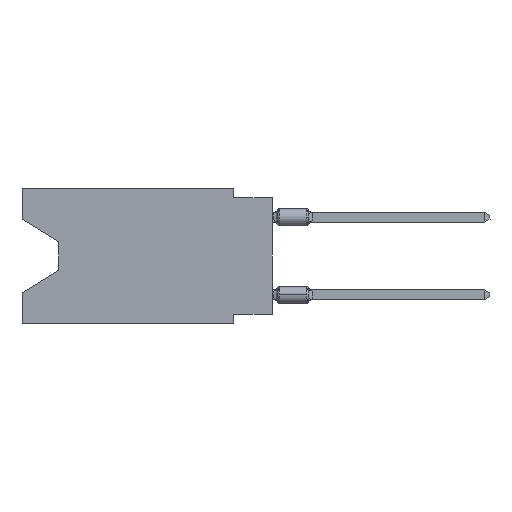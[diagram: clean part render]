
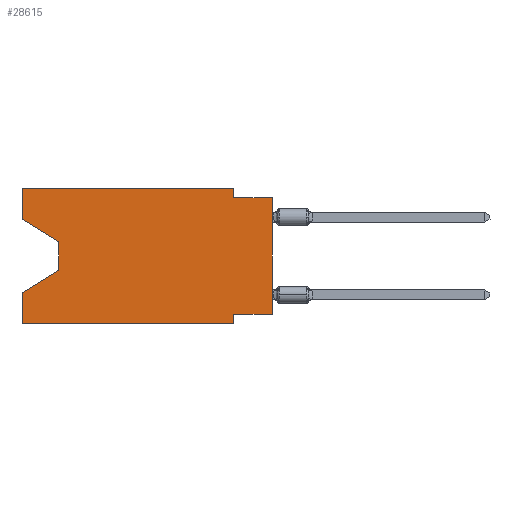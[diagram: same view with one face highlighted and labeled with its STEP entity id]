
A CAD part, left-side view. The second image highlights one B-rep face of the part: STEP entity #28615.
In plain terms, the highlighted planar face has unit normal (-1, 0, 0).
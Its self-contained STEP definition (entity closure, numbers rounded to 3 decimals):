
#139 = VERTEX_POINT ( 'NONE', #449 ) ;
#225 = DIRECTION ( 'NONE',  ( 0., 0.855, -0.519 ) ) ;
#449 = CARTESIAN_POINT ( 'NONE',  ( 0., 2.54, 0. ) ) ;
#458 = LINE ( 'NONE', #601, #13027 ) ;
#601 = CARTESIAN_POINT ( 'NONE',  ( 0., 2.54, -8.89 ) ) ;
#756 = VERTEX_POINT ( 'NONE', #26318 ) ;
#766 = DIRECTION ( 'NONE',  ( 0., -1., 0. ) ) ;
#1188 = CARTESIAN_POINT ( 'NONE',  ( 0., 16.383, -8.89 ) ) ;
#1565 = EDGE_CURVE ( 'NONE', #23276, #14872, #20340, .T. ) ;
#2100 = DIRECTION ( 'NONE',  ( 0., -1., 0. ) ) ;
#2121 = ORIENTED_EDGE ( 'NONE', *, *, #10918, .T. ) ;
#2343 = EDGE_LOOP ( 'NONE', ( #24505, #21543, #2121, #18915, #24399, #26511, #4750, #2411, #23506, #7458, #22411, #13040 ) ) ;
#2411 = ORIENTED_EDGE ( 'NONE', *, *, #8460, .T. ) ;
#2431 = CARTESIAN_POINT ( 'NONE',  ( 0., 13.97, -5.385 ) ) ;
#2976 = DIRECTION ( 'NONE',  ( 0., 0., 1. ) ) ;
#4326 = VERTEX_POINT ( 'NONE', #18522 ) ;
#4654 = CARTESIAN_POINT ( 'NONE',  ( 0., 16.383, 0. ) ) ;
#4750 = ORIENTED_EDGE ( 'NONE', *, *, #19683, .F. ) ;
#5405 = CARTESIAN_POINT ( 'NONE',  ( 0., 13.97, -3.505 ) ) ;
#5602 = LINE ( 'NONE', #7360, #12120 ) ;
#6143 = PLANE ( 'NONE',  #20646 ) ;
#6311 = VERTEX_POINT ( 'NONE', #9473 ) ;
#6478 = CARTESIAN_POINT ( 'NONE',  ( 0., 0., -0.635 ) ) ;
#6946 = LINE ( 'NONE', #2431, #7659 ) ;
#7360 = CARTESIAN_POINT ( 'NONE',  ( 0., 13.97, -3.505 ) ) ;
#7458 = ORIENTED_EDGE ( 'NONE', *, *, #9788, .F. ) ;
#7653 = CARTESIAN_POINT ( 'NONE',  ( 0., 0., -0.635 ) ) ;
#7659 = VECTOR ( 'NONE', #225, 1000. ) ;
#7799 = LINE ( 'NONE', #6478, #27815 ) ;
#8460 = EDGE_CURVE ( 'NONE', #4326, #24182, #16311, .T. ) ;
#8604 = CARTESIAN_POINT ( 'NONE',  ( 0., 16.383, -2.038 ) ) ;
#9473 = CARTESIAN_POINT ( 'NONE',  ( 0., 16.383, -2.038 ) ) ;
#9788 = EDGE_CURVE ( 'NONE', #139, #14506, #10714, .T. ) ;
#9971 = CARTESIAN_POINT ( 'NONE',  ( 0., 2.54, -8.89 ) ) ;
#10013 = DIRECTION ( 'NONE',  ( 0., -1., 0. ) ) ;
#10368 = DIRECTION ( 'NONE',  ( 0., -0.855, -0.519 ) ) ;
#10557 = DIRECTION ( 'NONE',  ( 0., 0., -1. ) ) ;
#10696 = DIRECTION ( 'NONE',  ( 0., 0., -1. ) ) ;
#10714 = LINE ( 'NONE', #14969, #21642 ) ;
#10918 = EDGE_CURVE ( 'NONE', #26119, #14872, #6946, .T. ) ;
#11070 = EDGE_CURVE ( 'NONE', #14506, #24182, #7799, .T. ) ;
#11800 = VECTOR ( 'NONE', #2976, 1000. ) ;
#12120 = VECTOR ( 'NONE', #12334, 1000. ) ;
#12334 = DIRECTION ( 'NONE',  ( 0., 0., -1. ) ) ;
#12480 = VECTOR ( 'NONE', #10013, 1000. ) ;
#12575 = VERTEX_POINT ( 'NONE', #9971 ) ;
#12742 = LINE ( 'NONE', #12884, #26695 ) ;
#12884 = CARTESIAN_POINT ( 'NONE',  ( 0., 0., -8.255 ) ) ;
#13008 = VECTOR ( 'NONE', #23690, 1000. ) ;
#13027 = VECTOR ( 'NONE', #14064, 1000. ) ;
#13040 = ORIENTED_EDGE ( 'NONE', *, *, #22760, .F. ) ;
#13622 = CARTESIAN_POINT ( 'NONE',  ( 0., 16.383, 0. ) ) ;
#14064 = DIRECTION ( 'NONE',  ( 0., 0., -1. ) ) ;
#14276 = EDGE_CURVE ( 'NONE', #14940, #139, #16785, .T. ) ;
#14506 = VERTEX_POINT ( 'NONE', #17365 ) ;
#14727 = LINE ( 'NONE', #24129, #13008 ) ;
#14858 = CARTESIAN_POINT ( 'NONE',  ( 0., 16.383, 0. ) ) ;
#14872 = VERTEX_POINT ( 'NONE', #22011 ) ;
#14940 = VERTEX_POINT ( 'NONE', #13622 ) ;
#14969 = CARTESIAN_POINT ( 'NONE',  ( 0., 2.54, 0. ) ) ;
#15074 = LINE ( 'NONE', #8604, #21384 ) ;
#15097 = CARTESIAN_POINT ( 'NONE',  ( 0., 16.383, 0. ) ) ;
#16311 = LINE ( 'NONE', #23073, #11800 ) ;
#16785 = LINE ( 'NONE', #14858, #12480 ) ;
#17012 = LINE ( 'NONE', #1188, #20180 ) ;
#17365 = CARTESIAN_POINT ( 'NONE',  ( 0., 2.54, -0.635 ) ) ;
#17693 = VECTOR ( 'NONE', #20053, 1000. ) ;
#18522 = CARTESIAN_POINT ( 'NONE',  ( 0., 0., -8.255 ) ) ;
#18915 = ORIENTED_EDGE ( 'NONE', *, *, #1565, .F. ) ;
#19431 = EDGE_CURVE ( 'NONE', #23276, #12575, #17012, .T. ) ;
#19648 = CARTESIAN_POINT ( 'NONE',  ( 0., 13.97, -5.385 ) ) ;
#19683 = EDGE_CURVE ( 'NONE', #4326, #756, #12742, .T. ) ;
#20053 = DIRECTION ( 'NONE',  ( 0., 0., 1. ) ) ;
#20180 = VECTOR ( 'NONE', #766, 1000. ) ;
#20340 = LINE ( 'NONE', #4654, #17693 ) ;
#20646 = AXIS2_PLACEMENT_3D ( 'NONE', #15097, #24052, #10696 ) ;
#21220 = EDGE_CURVE ( 'NONE', #6311, #25869, #15074, .T. ) ;
#21384 = VECTOR ( 'NONE', #10368, 1000. ) ;
#21543 = ORIENTED_EDGE ( 'NONE', *, *, #26731, .T. ) ;
#21642 = VECTOR ( 'NONE', #10557, 1000. ) ;
#22011 = CARTESIAN_POINT ( 'NONE',  ( 0., 16.383, -6.852 ) ) ;
#22411 = ORIENTED_EDGE ( 'NONE', *, *, #14276, .F. ) ;
#22760 = EDGE_CURVE ( 'NONE', #6311, #14940, #14727, .T. ) ;
#22881 = CARTESIAN_POINT ( 'NONE',  ( 0., 16.383, -8.89 ) ) ;
#23073 = CARTESIAN_POINT ( 'NONE',  ( 0., 0., 0. ) ) ;
#23205 = EDGE_CURVE ( 'NONE', #756, #12575, #458, .T. ) ;
#23276 = VERTEX_POINT ( 'NONE', #22881 ) ;
#23506 = ORIENTED_EDGE ( 'NONE', *, *, #11070, .F. ) ;
#23690 = DIRECTION ( 'NONE',  ( 0., 0., 1. ) ) ;
#24052 = DIRECTION ( 'NONE',  ( 1., 0., 0. ) ) ;
#24129 = CARTESIAN_POINT ( 'NONE',  ( 0., 16.383, 0. ) ) ;
#24182 = VERTEX_POINT ( 'NONE', #7653 ) ;
#24399 = ORIENTED_EDGE ( 'NONE', *, *, #19431, .T. ) ;
#24505 = ORIENTED_EDGE ( 'NONE', *, *, #21220, .T. ) ;
#24926 = DIRECTION ( 'NONE',  ( 0., 1., 0. ) ) ;
#25869 = VERTEX_POINT ( 'NONE', #5405 ) ;
#26119 = VERTEX_POINT ( 'NONE', #19648 ) ;
#26318 = CARTESIAN_POINT ( 'NONE',  ( 0., 2.54, -8.255 ) ) ;
#26511 = ORIENTED_EDGE ( 'NONE', *, *, #23205, .F. ) ;
#26695 = VECTOR ( 'NONE', #24926, 1000. ) ;
#26731 = EDGE_CURVE ( 'NONE', #25869, #26119, #5602, .T. ) ;
#27815 = VECTOR ( 'NONE', #2100, 1000. ) ;
#28450 = FACE_OUTER_BOUND ( 'NONE', #2343, .T. ) ;
#28615 = ADVANCED_FACE ( 'NONE', ( #28450 ), #6143, .F. ) ;
